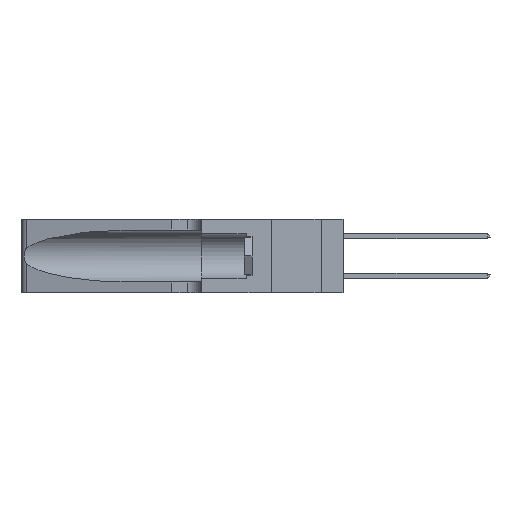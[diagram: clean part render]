
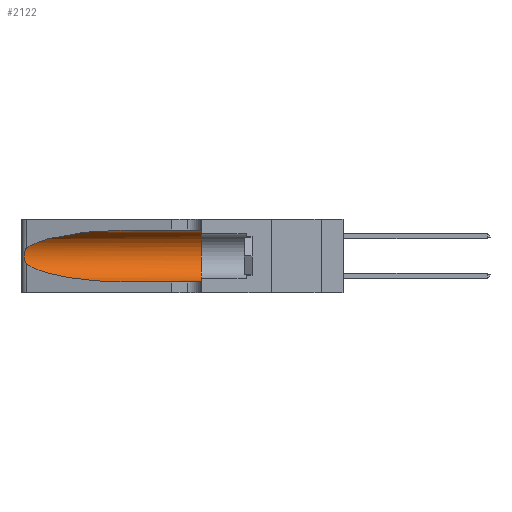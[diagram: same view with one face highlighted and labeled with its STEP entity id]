
A CAD part, left-side view. The second image highlights one B-rep face of the part: STEP entity #2122.
In plain terms, the highlighted cylindrical face has radius 3.308 mm (diameter 6.617 mm), a partial arc.
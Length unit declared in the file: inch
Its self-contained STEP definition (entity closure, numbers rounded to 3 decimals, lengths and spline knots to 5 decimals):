
#852 = DIRECTION ( 'NONE',  ( 0., -1., 0. ) ) ;
#1075 = EDGE_CURVE ( 'NONE', #26039, #14613, #15409, .T. ) ;
#1297 = CARTESIAN_POINT ( 'NONE',  ( 0.26075, 1.23896, 0.178 ) ) ;
#1403 = ORIENTED_EDGE ( 'NONE', *, *, #1631, .T. ) ;
#1631 = EDGE_CURVE ( 'NONE', #26039, #27591, #10026, .T. ) ;
#1859 = CARTESIAN_POINT ( 'NONE',  ( 0.25487, 1.22718, 0.22369 ) ) ;
#2122 = ADVANCED_FACE ( 'NONE', ( #3197 ), #2227, .F. ) ;
#2227 = CYLINDRICAL_SURFACE ( 'NONE', #4438, 0.13025 ) ;
#2464 = CARTESIAN_POINT ( 'NONE',  ( 0.1305, 0.35, 0.185 ) ) ;
#3197 = FACE_OUTER_BOUND ( 'NONE', #12880, .T. ) ;
#3479 = CARTESIAN_POINT ( 'NONE',  ( 0.1305, 0.35, 0.31525 ) ) ;
#4371 = CARTESIAN_POINT ( 'NONE',  ( 0.25856, 1.23593, 0.16098 ) ) ;
#4438 = AXIS2_PLACEMENT_3D ( 'NONE', #15641, #12547, #6291 ) ;
#5568 = DIRECTION ( 'NONE',  ( 0., 0., 1. ) ) ;
#6291 = DIRECTION ( 'NONE',  ( 0., 0., -1. ) ) ;
#7405 = CARTESIAN_POINT ( 'NONE',  ( 0.25555, 1.22994, 0.2215 ) ) ;
#7548 = CARTESIAN_POINT ( 'NONE',  ( 0.25639, 1.23186, 0.15144 ) ) ;
#7714 = CARTESIAN_POINT ( 'NONE',  ( 0.25487, 1.22718, 0.14631 ) ) ;
#8874 = ORIENTED_EDGE ( 'NONE', *, *, #1075, .F. ) ;
#10026 =( BOUNDED_CURVE ( )  B_SPLINE_CURVE ( 3, ( #13507, #16573, #37826, #19648 ),
 .UNSPECIFIED., .F., .T. ) 
 B_SPLINE_CURVE_WITH_KNOTS ( ( 4, 4 ),
 ( 1.5708, 2.84003 ),
 .UNSPECIFIED. ) 
 CURVE ( )  GEOMETRIC_REPRESENTATION_ITEM ( )  RATIONAL_B_SPLINE_CURVE ( ( 1., 0.87, 0.87, 1. ) ) 
 REPRESENTATION_ITEM ( '' )  );
#10501 = EDGE_CURVE ( 'NONE', #14613, #36096, #17915, .T. ) ;
#10666 = CARTESIAN_POINT ( 'NONE',  ( 0.25487, 1.22718, 0.14631 ) ) ;
#10835 = CARTESIAN_POINT ( 'NONE',  ( 0.18966, 0.96281, 0.05475 ) ) ;
#11255 = B_SPLINE_CURVE_WITH_KNOTS ( 'NONE', 3,
 ( #28789, #7405, #13641, #34932, #16706, #37960, #19765, #1297, #22823, #4371, #25877, #7548, #28929, #10666 ),
 .UNSPECIFIED., .F., .F.,
 ( 4, 2, 2, 2, 2, 2, 4 ),
 ( 0., 0.00027, 0.00053, 0.00107, 0.0016, 0.00187, 0.00214 ),
 .UNSPECIFIED. ) ;
#12547 = DIRECTION ( 'NONE',  ( 0., -1., 0. ) ) ;
#12802 = CARTESIAN_POINT ( 'NONE',  ( 0.1305, 0.72297, 0.31525 ) ) ;
#12880 = EDGE_LOOP ( 'NONE', ( #1403, #35257, #23854, #20324, #15286, #8874 ) ) ;
#13402 = VECTOR ( 'NONE', #852, 39.37008 ) ;
#13507 = CARTESIAN_POINT ( 'NONE',  ( 0.1305, 0.72297, 0.31525 ) ) ;
#13641 = CARTESIAN_POINT ( 'NONE',  ( 0.25639, 1.23184, 0.21858 ) ) ;
#13748 = AXIS2_PLACEMENT_3D ( 'NONE', #2464, #23985, #5568 ) ;
#14406 = LINE ( 'NONE', #28360, #13402 ) ;
#14613 = VERTEX_POINT ( 'NONE', #3479 ) ;
#14762 = VERTEX_POINT ( 'NONE', #31864 ) ;
#15084 = CARTESIAN_POINT ( 'NONE',  ( 0.25487, 1.22718, 0.14631 ) ) ;
#15286 = ORIENTED_EDGE ( 'NONE', *, *, #10501, .F. ) ;
#15409 = LINE ( 'NONE', #23283, #38684 ) ;
#15641 = CARTESIAN_POINT ( 'NONE',  ( 0.1305, 1.61858, 0.185 ) ) ;
#16573 = CARTESIAN_POINT ( 'NONE',  ( 0.18966, 0.96281, 0.31525 ) ) ;
#16706 = CARTESIAN_POINT ( 'NONE',  ( 0.25854, 1.2359, 0.20912 ) ) ;
#17915 = CIRCLE ( 'NONE', #13748, 0.13025 ) ;
#18996 = CARTESIAN_POINT ( 'NONE',  ( 0.1305, 0.35, 0.05475 ) ) ;
#19648 = CARTESIAN_POINT ( 'NONE',  ( 0.25487, 1.22718, 0.22369 ) ) ;
#19765 = CARTESIAN_POINT ( 'NONE',  ( 0.26075, 1.23896, 0.19203 ) ) ;
#20227 = DIRECTION ( 'NONE',  ( 0., -1., 0. ) ) ;
#20324 = ORIENTED_EDGE ( 'NONE', *, *, #33522, .T. ) ;
#22823 = CARTESIAN_POINT ( 'NONE',  ( 0.26017, 1.23833, 0.17102 ) ) ;
#23283 = CARTESIAN_POINT ( 'NONE',  ( 0.1305, 1.61858, 0.31525 ) ) ;
#23714 = EDGE_CURVE ( 'NONE', #37060, #14762, #39569, .T. ) ;
#23854 = ORIENTED_EDGE ( 'NONE', *, *, #23714, .T. ) ;
#23985 = DIRECTION ( 'NONE',  ( 0., 1., 0. ) ) ;
#25877 = CARTESIAN_POINT ( 'NONE',  ( 0.25789, 1.23486, 0.15765 ) ) ;
#26039 = VERTEX_POINT ( 'NONE', #12802 ) ;
#26044 = CARTESIAN_POINT ( 'NONE',  ( 0.2373, 1.15595, 0.08982 ) ) ;
#27591 = VERTEX_POINT ( 'NONE', #1859 ) ;
#28360 = CARTESIAN_POINT ( 'NONE',  ( 0.1305, 1.61858, 0.05475 ) ) ;
#28789 = CARTESIAN_POINT ( 'NONE',  ( 0.25487, 1.22718, 0.22369 ) ) ;
#28929 = CARTESIAN_POINT ( 'NONE',  ( 0.25555, 1.22993, 0.14849 ) ) ;
#31864 = CARTESIAN_POINT ( 'NONE',  ( 0.1305, 0.72297, 0.05475 ) ) ;
#32183 = CARTESIAN_POINT ( 'NONE',  ( 0.1305, 0.72297, 0.05475 ) ) ;
#33522 = EDGE_CURVE ( 'NONE', #14762, #36096, #14406, .T. ) ;
#34932 = CARTESIAN_POINT ( 'NONE',  ( 0.25787, 1.23484, 0.2124 ) ) ;
#35257 = ORIENTED_EDGE ( 'NONE', *, *, #36228, .T. ) ;
#36096 = VERTEX_POINT ( 'NONE', #18996 ) ;
#36228 = EDGE_CURVE ( 'NONE', #27591, #37060, #11255, .T. ) ;
#37060 = VERTEX_POINT ( 'NONE', #15084 ) ;
#37826 = CARTESIAN_POINT ( 'NONE',  ( 0.2373, 1.15595, 0.28018 ) ) ;
#37960 = CARTESIAN_POINT ( 'NONE',  ( 0.26018, 1.23835, 0.19895 ) ) ;
#38684 = VECTOR ( 'NONE', #20227, 39.37008 ) ;
#39569 =( BOUNDED_CURVE ( )  B_SPLINE_CURVE ( 3, ( #7714, #26044, #10835, #32183 ),
 .UNSPECIFIED., .F., .T. ) 
 B_SPLINE_CURVE_WITH_KNOTS ( ( 4, 4 ),
 ( 3.44316, 4.71239 ),
 .UNSPECIFIED. ) 
 CURVE ( )  GEOMETRIC_REPRESENTATION_ITEM ( )  RATIONAL_B_SPLINE_CURVE ( ( 1., 0.87, 0.87, 1. ) ) 
 REPRESENTATION_ITEM ( '' )  );
